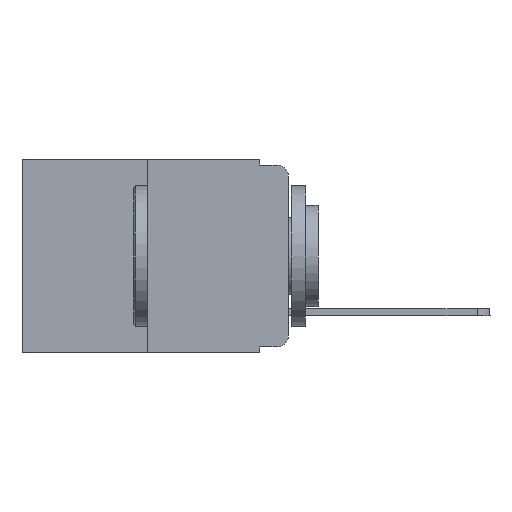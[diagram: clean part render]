
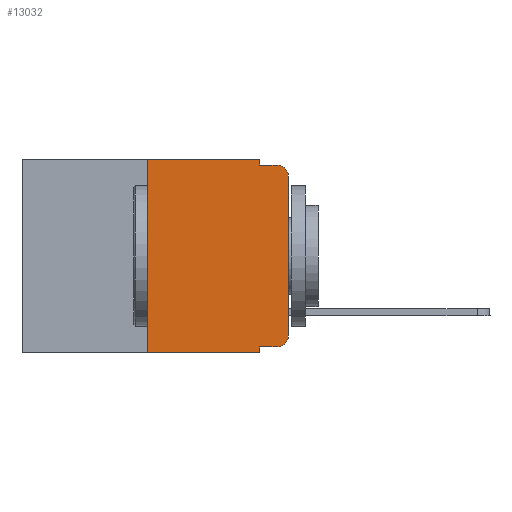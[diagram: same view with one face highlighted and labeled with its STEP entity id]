
A CAD part, left-side view. The second image highlights one B-rep face of the part: STEP entity #13032.
In plain terms, the highlighted planar face has unit normal (-1, 0, 0).
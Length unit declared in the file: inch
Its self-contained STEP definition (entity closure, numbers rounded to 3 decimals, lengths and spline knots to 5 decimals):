
#251 = CARTESIAN_POINT ( 'NONE',  ( 0., 0., -0.313 ) ) ;
#272 = DIRECTION ( 'NONE',  ( 0., -1., 0. ) ) ;
#396 = CARTESIAN_POINT ( 'NONE',  ( 0., 0.051, 0. ) ) ;
#954 = LINE ( 'NONE', #14791, #11136 ) ;
#1101 = DIRECTION ( 'NONE',  ( 0., -1., 0. ) ) ;
#1400 = AXIS2_PLACEMENT_3D ( 'NONE', #9194, #14525, #6392 ) ;
#1967 = DIRECTION ( 'NONE',  ( 0., 0., -1. ) ) ;
#2141 = DIRECTION ( 'NONE',  ( 0., 0., -1. ) ) ;
#2521 = EDGE_CURVE ( 'NONE', #13241, #16175, #2632, .T. ) ;
#2632 = LINE ( 'NONE', #8602, #7847 ) ;
#2738 = EDGE_LOOP ( 'NONE', ( #15093, #13298, #16491, #2820, #13436, #12557, #16555, #7554, #5999, #17388 ) ) ;
#2782 = VERTEX_POINT ( 'NONE', #11470 ) ;
#2820 = ORIENTED_EDGE ( 'NONE', *, *, #5189, .F. ) ;
#3084 = EDGE_CURVE ( 'NONE', #2782, #14812, #12368, .T. ) ;
#3362 = CIRCLE ( 'NONE', #15664, 0.02 ) ;
#3431 = EDGE_CURVE ( 'NONE', #14140, #5288, #11044, .T. ) ;
#3637 = DIRECTION ( 'NONE',  ( 0., -1., 0. ) ) ;
#3944 = CARTESIAN_POINT ( 'NONE',  ( 0., 0.02, -0.01 ) ) ;
#4142 = VECTOR ( 'NONE', #272, 39.37008 ) ;
#4560 = VECTOR ( 'NONE', #1101, 39.37008 ) ;
#5189 = EDGE_CURVE ( 'NONE', #14020, #15109, #12289, .T. ) ;
#5288 = VERTEX_POINT ( 'NONE', #8911 ) ;
#5360 = LINE ( 'NONE', #17779, #14897 ) ;
#5808 = DIRECTION ( 'NONE',  ( 0., -1., 0. ) ) ;
#5999 = ORIENTED_EDGE ( 'NONE', *, *, #3084, .T. ) ;
#6049 = VECTOR ( 'NONE', #13141, 39.37008 ) ;
#6331 = CARTESIAN_POINT ( 'NONE',  ( 0., 0.473, 0. ) ) ;
#6392 = DIRECTION ( 'NONE',  ( 0., 0., -1. ) ) ;
#6804 = EDGE_CURVE ( 'NONE', #15143, #14020, #7375, .T. ) ;
#7359 = VECTOR ( 'NONE', #13193, 39.37008 ) ;
#7375 = LINE ( 'NONE', #15465, #4142 ) ;
#7469 = DIRECTION ( 'NONE',  ( -1., 0., 0. ) ) ;
#7554 = ORIENTED_EDGE ( 'NONE', *, *, #17115, .F. ) ;
#7847 = VECTOR ( 'NONE', #5808, 39.37008 ) ;
#8082 = DIRECTION ( 'NONE',  ( 0., 0., 1. ) ) ;
#8137 = FACE_OUTER_BOUND ( 'NONE', #2738, .T. ) ;
#8602 = CARTESIAN_POINT ( 'NONE',  ( 0., 0.473, -0.343 ) ) ;
#8911 = CARTESIAN_POINT ( 'NONE',  ( 0., 0., -0.03 ) ) ;
#8985 = CARTESIAN_POINT ( 'NONE',  ( 0., 0.02, -0.333 ) ) ;
#9077 = DIRECTION ( 'NONE',  ( 1., 0., 0. ) ) ;
#9194 = CARTESIAN_POINT ( 'NONE',  ( 0., 0.02, -0.313 ) ) ;
#9279 = EDGE_CURVE ( 'NONE', #13241, #15143, #5360, .T. ) ;
#9486 = CARTESIAN_POINT ( 'NONE',  ( 0., 0.051, -0.333 ) ) ;
#9699 = EDGE_CURVE ( 'NONE', #14812, #14140, #11834, .T. ) ;
#10129 = VECTOR ( 'NONE', #11330, 39.37008 ) ;
#10146 = EDGE_CURVE ( 'NONE', #5288, #12043, #3362, .T. ) ;
#10242 = CARTESIAN_POINT ( 'NONE',  ( 0., 0., 0. ) ) ;
#10346 = EDGE_CURVE ( 'NONE', #15109, #12043, #954, .T. ) ;
#10375 = AXIS2_PLACEMENT_3D ( 'NONE', #6331, #9077, #2141 ) ;
#10568 = PLANE ( 'NONE',  #10375 ) ;
#11044 = LINE ( 'NONE', #10242, #7359 ) ;
#11136 = VECTOR ( 'NONE', #3637, 39.37008 ) ;
#11330 = DIRECTION ( 'NONE',  ( 0., 0., -1. ) ) ;
#11470 = CARTESIAN_POINT ( 'NONE',  ( 0., 0.051, -0.333 ) ) ;
#11834 = CIRCLE ( 'NONE', #1400, 0.02 ) ;
#12043 = VERTEX_POINT ( 'NONE', #3944 ) ;
#12130 = LINE ( 'NONE', #17155, #6049 ) ;
#12289 = LINE ( 'NONE', #16835, #10129 ) ;
#12368 = LINE ( 'NONE', #9486, #4560 ) ;
#12557 = ORIENTED_EDGE ( 'NONE', *, *, #9279, .F. ) ;
#13032 = ADVANCED_FACE ( 'NONE', ( #8137 ), #10568, .F. ) ;
#13048 = CARTESIAN_POINT ( 'NONE',  ( 0., 0.02, -0.03 ) ) ;
#13141 = DIRECTION ( 'NONE',  ( 0., 0., -1. ) ) ;
#13177 = CARTESIAN_POINT ( 'NONE',  ( 0., 0.25, -0.343 ) ) ;
#13193 = DIRECTION ( 'NONE',  ( 0., 0., 1. ) ) ;
#13241 = VERTEX_POINT ( 'NONE', #13177 ) ;
#13298 = ORIENTED_EDGE ( 'NONE', *, *, #10146, .T. ) ;
#13436 = ORIENTED_EDGE ( 'NONE', *, *, #6804, .F. ) ;
#13723 = CARTESIAN_POINT ( 'NONE',  ( 0., 0.051, -0.01 ) ) ;
#14020 = VERTEX_POINT ( 'NONE', #396 ) ;
#14140 = VERTEX_POINT ( 'NONE', #251 ) ;
#14525 = DIRECTION ( 'NONE',  ( -1., 0., 0. ) ) ;
#14791 = CARTESIAN_POINT ( 'NONE',  ( 0., 0.051, -0.01 ) ) ;
#14812 = VERTEX_POINT ( 'NONE', #8985 ) ;
#14897 = VECTOR ( 'NONE', #8082, 39.37008 ) ;
#15093 = ORIENTED_EDGE ( 'NONE', *, *, #3431, .T. ) ;
#15109 = VERTEX_POINT ( 'NONE', #13723 ) ;
#15143 = VERTEX_POINT ( 'NONE', #16523 ) ;
#15465 = CARTESIAN_POINT ( 'NONE',  ( 0., 0.473, 0. ) ) ;
#15664 = AXIS2_PLACEMENT_3D ( 'NONE', #13048, #7469, #1967 ) ;
#16175 = VERTEX_POINT ( 'NONE', #16525 ) ;
#16491 = ORIENTED_EDGE ( 'NONE', *, *, #10346, .F. ) ;
#16523 = CARTESIAN_POINT ( 'NONE',  ( 0., 0.25, 0. ) ) ;
#16525 = CARTESIAN_POINT ( 'NONE',  ( 0., 0.051, -0.343 ) ) ;
#16555 = ORIENTED_EDGE ( 'NONE', *, *, #2521, .T. ) ;
#16835 = CARTESIAN_POINT ( 'NONE',  ( 0., 0.051, 0. ) ) ;
#17115 = EDGE_CURVE ( 'NONE', #2782, #16175, #12130, .T. ) ;
#17155 = CARTESIAN_POINT ( 'NONE',  ( 0., 0.051, 0. ) ) ;
#17388 = ORIENTED_EDGE ( 'NONE', *, *, #9699, .T. ) ;
#17779 = CARTESIAN_POINT ( 'NONE',  ( 0., 0.25, 0. ) ) ;
